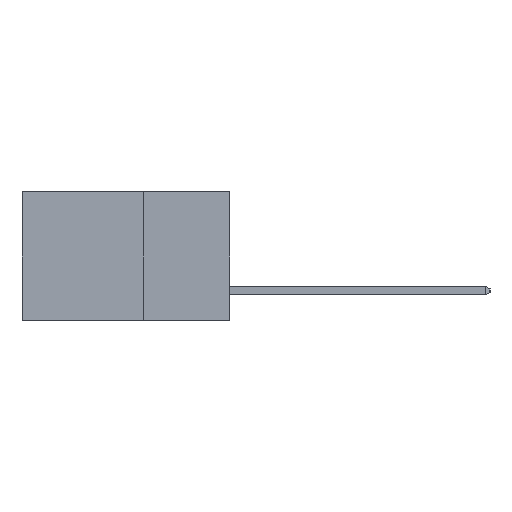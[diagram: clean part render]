
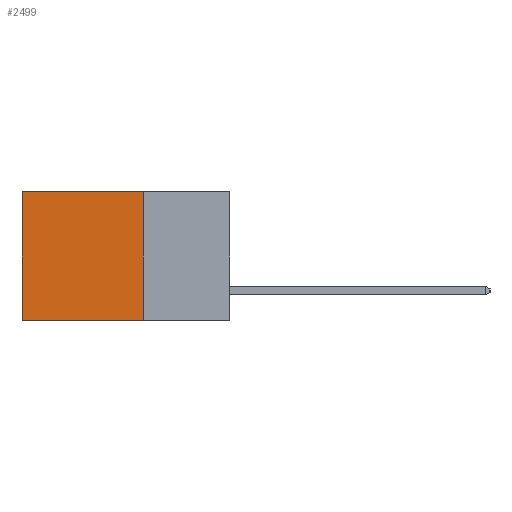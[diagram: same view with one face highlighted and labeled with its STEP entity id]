
A CAD part, left-side view. The second image highlights one B-rep face of the part: STEP entity #2499.
In plain terms, the highlighted planar face has unit normal (-1, 0, 0).
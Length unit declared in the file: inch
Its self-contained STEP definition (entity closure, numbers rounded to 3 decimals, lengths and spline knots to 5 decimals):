
#278 = DIRECTION ( 'NONE',  ( 0., 0., -1. ) ) ;
#729 = LINE ( 'NONE', #5663, #1906 ) ;
#875 = VECTOR ( 'NONE', #8602, 39.37008 ) ;
#989 = CARTESIAN_POINT ( 'NONE',  ( 0.2615, 0.6, 0. ) ) ;
#1388 = PLANE ( 'NONE',  #5072 ) ;
#1500 = EDGE_CURVE ( 'NONE', #10936, #5667, #5151, .T. ) ;
#1848 = CARTESIAN_POINT ( 'NONE',  ( 0.2615, 0.6, -0.37 ) ) ;
#1906 = VECTOR ( 'NONE', #13338, 39.37008 ) ;
#2499 = ADVANCED_FACE ( 'NONE', ( #9367 ), #1388, .F. ) ;
#2655 = DIRECTION ( 'NONE',  ( 0., 1., 0. ) ) ;
#3328 = EDGE_CURVE ( 'NONE', #9544, #10184, #729, .T. ) ;
#3747 = EDGE_CURVE ( 'NONE', #10936, #9544, #3955, .T. ) ;
#3765 = VECTOR ( 'NONE', #7573, 39.37008 ) ;
#3869 = CARTESIAN_POINT ( 'NONE',  ( 0.2615, 0.25, -0.37 ) ) ;
#3955 = LINE ( 'NONE', #14022, #875 ) ;
#4640 = CARTESIAN_POINT ( 'NONE',  ( 0.2615, 0.25, -0.37 ) ) ;
#5072 = AXIS2_PLACEMENT_3D ( 'NONE', #4640, #7826, #278 ) ;
#5151 = LINE ( 'NONE', #10796, #3765 ) ;
#5332 = EDGE_LOOP ( 'NONE', ( #11420, #11919, #14069, #12012 ) ) ;
#5663 = CARTESIAN_POINT ( 'NONE',  ( 0.2615, 0.6, -0.37 ) ) ;
#5667 = VERTEX_POINT ( 'NONE', #3869 ) ;
#7573 = DIRECTION ( 'NONE',  ( 0., 0., -1. ) ) ;
#7826 = DIRECTION ( 'NONE',  ( 1., 0., 0. ) ) ;
#8602 = DIRECTION ( 'NONE',  ( 0., 1., 0. ) ) ;
#8943 = LINE ( 'NONE', #9868, #10803 ) ;
#9367 = FACE_OUTER_BOUND ( 'NONE', #5332, .T. ) ;
#9544 = VERTEX_POINT ( 'NONE', #989 ) ;
#9868 = CARTESIAN_POINT ( 'NONE',  ( 0.2615, 0.25, -0.37 ) ) ;
#10184 = VERTEX_POINT ( 'NONE', #1848 ) ;
#10796 = CARTESIAN_POINT ( 'NONE',  ( 0.2615, 0.25, -0.37 ) ) ;
#10803 = VECTOR ( 'NONE', #2655, 39.37008 ) ;
#10936 = VERTEX_POINT ( 'NONE', #13637 ) ;
#11420 = ORIENTED_EDGE ( 'NONE', *, *, #3328, .T. ) ;
#11819 = EDGE_CURVE ( 'NONE', #5667, #10184, #8943, .T. ) ;
#11919 = ORIENTED_EDGE ( 'NONE', *, *, #11819, .F. ) ;
#12012 = ORIENTED_EDGE ( 'NONE', *, *, #3747, .T. ) ;
#13338 = DIRECTION ( 'NONE',  ( 0., 0., -1. ) ) ;
#13637 = CARTESIAN_POINT ( 'NONE',  ( 0.2615, 0.25, 0. ) ) ;
#14022 = CARTESIAN_POINT ( 'NONE',  ( 0.2615, 0.25, 0. ) ) ;
#14069 = ORIENTED_EDGE ( 'NONE', *, *, #1500, .F. ) ;
